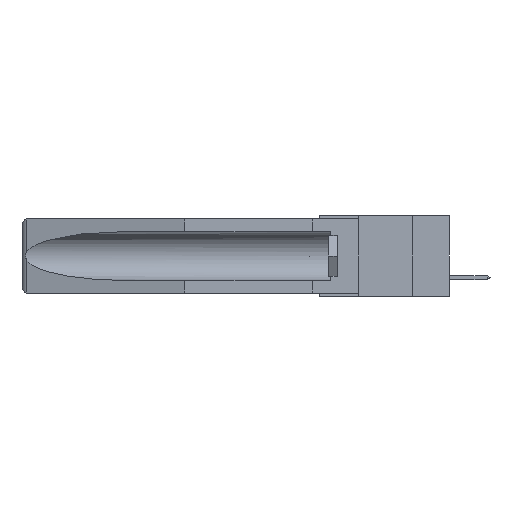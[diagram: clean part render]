
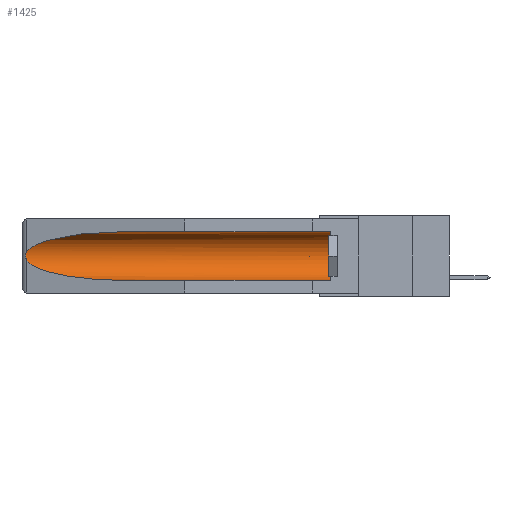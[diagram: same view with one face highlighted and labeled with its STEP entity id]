
A CAD part, left-side view. The second image highlights one B-rep face of the part: STEP entity #1425.
In plain terms, the highlighted cylindrical face has radius 2.857 mm (diameter 5.715 mm), a partial arc.
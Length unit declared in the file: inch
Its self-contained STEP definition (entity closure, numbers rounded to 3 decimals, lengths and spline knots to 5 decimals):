
#1090 = ORIENTED_EDGE ( 'NONE', *, *, #17143, .T. ) ;
#1425 = ADVANCED_FACE ( 'NONE', ( #10832 ), #3818, .F. ) ;
#1811 = ORIENTED_EDGE ( 'NONE', *, *, #33118, .T. ) ;
#2207 = CARTESIAN_POINT ( 'NONE',  ( 0.2673, 1.5327, -0.16383 ) ) ;
#2224 = DIRECTION ( 'NONE',  ( 0., 1., 0. ) ) ;
#2300 = CIRCLE ( 'NONE', #21425, 0.1125 ) ;
#2345 = VECTOR ( 'NONE', #2224, 39.37008 ) ;
#3818 = CYLINDRICAL_SURFACE ( 'NONE', #10970, 0.1125 ) ;
#3884 = EDGE_CURVE ( 'NONE', #24761, #12634, #32510, .T. ) ;
#4900 = ORIENTED_EDGE ( 'NONE', *, *, #10518, .T. ) ;
#5972 = CARTESIAN_POINT ( 'NONE',  ( 0.155, 0.126, -0.1715 ) ) ;
#7207 = CARTESIAN_POINT ( 'NONE',  ( 0.26597, 1.5296, -0.19026 ) ) ;
#10349 = VERTEX_POINT ( 'NONE', #29643 ) ;
#10518 = EDGE_CURVE ( 'NONE', #10349, #26888, #29194, .T. ) ;
#10832 = FACE_OUTER_BOUND ( 'NONE', #29835, .T. ) ;
#10970 = AXIS2_PLACEMENT_3D ( 'NONE', #24789, #19410, #17210 ) ;
#11248 = DIRECTION ( 'NONE',  ( 0., 0., 1. ) ) ;
#11552 = VERTEX_POINT ( 'NONE', #25414 ) ;
#12087 = DIRECTION ( 'NONE',  ( 0., 1., 0. ) ) ;
#12304 = CARTESIAN_POINT ( 'NONE',  ( 0.155, 1.07973, -0.059 ) ) ;
#12407 = CARTESIAN_POINT ( 'NONE',  ( 0.26537, 1.52718, -0.14972 ) ) ;
#12634 = VERTEX_POINT ( 'NONE', #31295 ) ;
#12852 =( BOUNDED_CURVE ( )  B_SPLINE_CURVE ( 3, ( #12304, #17836, #22919, #12407 ),
 .UNSPECIFIED., .F., .F. ) 
 B_SPLINE_CURVE_WITH_KNOTS ( ( 4, 4 ),
 ( 4.71239, 6.08839 ),
 .UNSPECIFIED. ) 
 CURVE ( )  GEOMETRIC_REPRESENTATION_ITEM ( )  RATIONAL_B_SPLINE_CURVE ( ( 1., 0.848, 0.848, 1. ) ) 
 REPRESENTATION_ITEM ( '' )  );
#13063 = CARTESIAN_POINT ( 'NONE',  ( 0.26537, 1.52718, -0.19328 ) ) ;
#15350 = ORIENTED_EDGE ( 'NONE', *, *, #20062, .T. ) ;
#15419 = CARTESIAN_POINT ( 'NONE',  ( 0.2675, 1.53308, -0.16763 ) ) ;
#16654 = CARTESIAN_POINT ( 'NONE',  ( 0.26537, 1.52718, -0.19328 ) ) ;
#17143 = EDGE_CURVE ( 'NONE', #26888, #12634, #23104, .T. ) ;
#17193 = ORIENTED_EDGE ( 'NONE', *, *, #27714, .T. ) ;
#17210 = DIRECTION ( 'NONE',  ( 0., 0., 1. ) ) ;
#17836 = CARTESIAN_POINT ( 'NONE',  ( 0.21114, 1.30732, -0.059 ) ) ;
#17928 = LINE ( 'NONE', #33487, #2345 ) ;
#19410 = DIRECTION ( 'NONE',  ( 0., 1., 0. ) ) ;
#20062 = EDGE_CURVE ( 'NONE', #11552, #20157, #17928, .T. ) ;
#20157 = VERTEX_POINT ( 'NONE', #20467 ) ;
#20328 = CARTESIAN_POINT ( 'NONE',  ( 0.2673, 1.53269, -0.17917 ) ) ;
#20467 = CARTESIAN_POINT ( 'NONE',  ( 0.155, 1.07973, -0.059 ) ) ;
#21377 = ORIENTED_EDGE ( 'NONE', *, *, #3884, .F. ) ;
#21425 = AXIS2_PLACEMENT_3D ( 'NONE', #5972, #24268, #11248 ) ;
#21484 = CARTESIAN_POINT ( 'NONE',  ( 0.25451, 1.48313, -0.24835 ) ) ;
#22873 = CARTESIAN_POINT ( 'NONE',  ( 0.26654, 1.53092, -0.15636 ) ) ;
#22919 = CARTESIAN_POINT ( 'NONE',  ( 0.25451, 1.48313, -0.09465 ) ) ;
#23104 =( BOUNDED_CURVE ( )  B_SPLINE_CURVE ( 3, ( #13063, #21484, #31751, #29174 ),
 .UNSPECIFIED., .F., .F. ) 
 B_SPLINE_CURVE_WITH_KNOTS ( ( 4, 4 ),
 ( 0.1948, 1.5708 ),
 .UNSPECIFIED. ) 
 CURVE ( )  GEOMETRIC_REPRESENTATION_ITEM ( )  RATIONAL_B_SPLINE_CURVE ( ( 1., 0.848, 0.848, 1. ) ) 
 REPRESENTATION_ITEM ( '' )  );
#24268 = DIRECTION ( 'NONE',  ( 0., -1., 0. ) ) ;
#24761 = VERTEX_POINT ( 'NONE', #30088 ) ;
#24789 = CARTESIAN_POINT ( 'NONE',  ( 0.155, -0.30754, -0.1715 ) ) ;
#24876 = CARTESIAN_POINT ( 'NONE',  ( 0.155, -0.30754, -0.284 ) ) ;
#25414 = CARTESIAN_POINT ( 'NONE',  ( 0.155, 0.126, -0.059 ) ) ;
#26888 = VERTEX_POINT ( 'NONE', #16654 ) ;
#27714 = EDGE_CURVE ( 'NONE', #20157, #10349, #12852, .T. ) ;
#28475 = CARTESIAN_POINT ( 'NONE',  ( 0.2675, 1.53308, -0.17534 ) ) ;
#28888 = VECTOR ( 'NONE', #12087, 39.37008 ) ;
#29174 = CARTESIAN_POINT ( 'NONE',  ( 0.155, 1.07973, -0.284 ) ) ;
#29194 = B_SPLINE_CURVE_WITH_KNOTS ( 'NONE', 3,
 ( #33465, #33579, #22873, #2207, #15419, #28475, #20328, #33345, #7207, #33241 ),
 .UNSPECIFIED., .F., .F.,
 ( 4, 2, 2, 2, 4 ),
 ( 0., 0.00029, 0.00058, 0.00087, 0.00117 ),
 .UNSPECIFIED. ) ;
#29643 = CARTESIAN_POINT ( 'NONE',  ( 0.26537, 1.52718, -0.14972 ) ) ;
#29835 = EDGE_LOOP ( 'NONE', ( #17193, #4900, #1090, #21377, #1811, #15350 ) ) ;
#30088 = CARTESIAN_POINT ( 'NONE',  ( 0.155, 0.126, -0.284 ) ) ;
#31295 = CARTESIAN_POINT ( 'NONE',  ( 0.155, 1.07973, -0.284 ) ) ;
#31751 = CARTESIAN_POINT ( 'NONE',  ( 0.21114, 1.30732, -0.284 ) ) ;
#32510 = LINE ( 'NONE', #24876, #28888 ) ;
#33118 = EDGE_CURVE ( 'NONE', #24761, #11552, #2300, .T. ) ;
#33241 = CARTESIAN_POINT ( 'NONE',  ( 0.26537, 1.52718, -0.19328 ) ) ;
#33345 = CARTESIAN_POINT ( 'NONE',  ( 0.26655, 1.53094, -0.18657 ) ) ;
#33465 = CARTESIAN_POINT ( 'NONE',  ( 0.26537, 1.52718, -0.14972 ) ) ;
#33487 = CARTESIAN_POINT ( 'NONE',  ( 0.155, -0.30754, -0.059 ) ) ;
#33579 = CARTESIAN_POINT ( 'NONE',  ( 0.26597, 1.52961, -0.15275 ) ) ;
